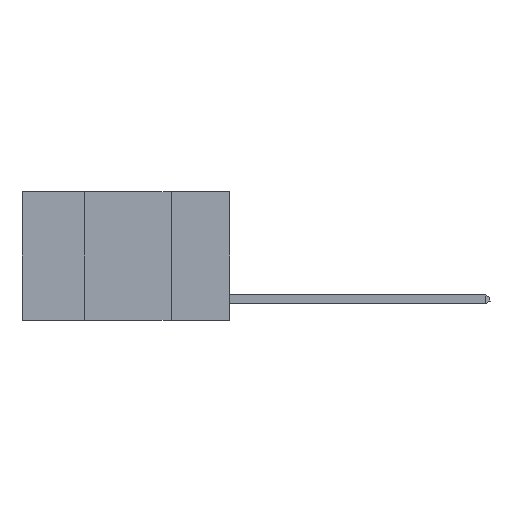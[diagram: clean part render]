
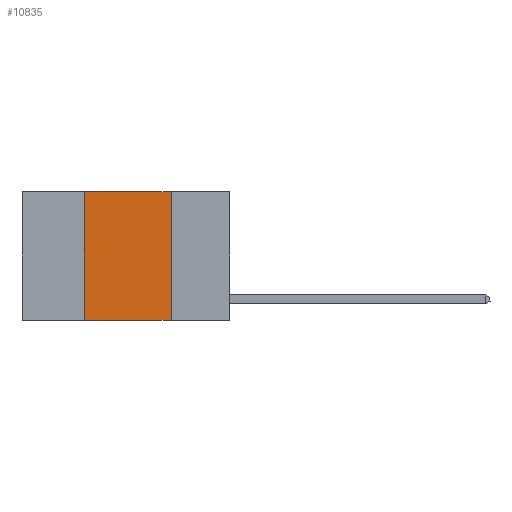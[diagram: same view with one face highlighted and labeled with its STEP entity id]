
A CAD part, left-side view. The second image highlights one B-rep face of the part: STEP entity #10835.
In plain terms, the highlighted planar face has unit normal (-1, 0, 0).
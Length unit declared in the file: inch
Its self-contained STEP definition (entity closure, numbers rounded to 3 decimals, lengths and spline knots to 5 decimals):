
#123 = CARTESIAN_POINT ( 'NONE',  ( 0., 0.17, 0. ) ) ;
#446 = ORIENTED_EDGE ( 'NONE', *, *, #1278, .F. ) ;
#529 = CARTESIAN_POINT ( 'NONE',  ( 0., 0.42, 0. ) ) ;
#716 = VERTEX_POINT ( 'NONE', #12476 ) ;
#964 = PLANE ( 'NONE',  #11970 ) ;
#1032 = CARTESIAN_POINT ( 'NONE',  ( 0., 0.6, 0. ) ) ;
#1186 = DIRECTION ( 'NONE',  ( 0., 0., -1. ) ) ;
#1278 = EDGE_CURVE ( 'NONE', #1766, #716, #4269, .T. ) ;
#1310 = VECTOR ( 'NONE', #12423, 39.37008 ) ;
#1478 = LINE ( 'NONE', #5616, #7635 ) ;
#1766 = VERTEX_POINT ( 'NONE', #123 ) ;
#2353 = DIRECTION ( 'NONE',  ( 0., -1., 0. ) ) ;
#2538 = EDGE_CURVE ( 'NONE', #12508, #716, #1478, .T. ) ;
#2647 = LINE ( 'NONE', #529, #10635 ) ;
#2713 = ORIENTED_EDGE ( 'NONE', *, *, #2538, .T. ) ;
#4038 = LINE ( 'NONE', #10348, #1310 ) ;
#4269 = LINE ( 'NONE', #8403, #6740 ) ;
#4941 = CARTESIAN_POINT ( 'NONE',  ( 0., 0.42, -0.37 ) ) ;
#5616 = CARTESIAN_POINT ( 'NONE',  ( 0., 0.6, -0.37 ) ) ;
#6150 = DIRECTION ( 'NONE',  ( 0., 0., -1. ) ) ;
#6703 = EDGE_LOOP ( 'NONE', ( #446, #7013, #10776, #2713 ) ) ;
#6740 = VECTOR ( 'NONE', #1186, 39.37008 ) ;
#7013 = ORIENTED_EDGE ( 'NONE', *, *, #10870, .F. ) ;
#7635 = VECTOR ( 'NONE', #2353, 39.37008 ) ;
#8403 = CARTESIAN_POINT ( 'NONE',  ( 0., 0.17, 0. ) ) ;
#10004 = DIRECTION ( 'NONE',  ( 0., 0., 1. ) ) ;
#10348 = CARTESIAN_POINT ( 'NONE',  ( 0., 0.6, 0. ) ) ;
#10635 = VECTOR ( 'NONE', #10004, 39.37008 ) ;
#10776 = ORIENTED_EDGE ( 'NONE', *, *, #11147, .F. ) ;
#10835 = ADVANCED_FACE ( 'NONE', ( #12624 ), #964, .F. ) ;
#10870 = EDGE_CURVE ( 'NONE', #11481, #1766, #4038, .T. ) ;
#11147 = EDGE_CURVE ( 'NONE', #12508, #11481, #2647, .T. ) ;
#11481 = VERTEX_POINT ( 'NONE', #12888 ) ;
#11970 = AXIS2_PLACEMENT_3D ( 'NONE', #1032, #12360, #6150 ) ;
#12360 = DIRECTION ( 'NONE',  ( 1., 0., 0. ) ) ;
#12423 = DIRECTION ( 'NONE',  ( 0., -1., 0. ) ) ;
#12476 = CARTESIAN_POINT ( 'NONE',  ( 0., 0.17, -0.37 ) ) ;
#12508 = VERTEX_POINT ( 'NONE', #4941 ) ;
#12624 = FACE_OUTER_BOUND ( 'NONE', #6703, .T. ) ;
#12888 = CARTESIAN_POINT ( 'NONE',  ( 0., 0.42, 0. ) ) ;
